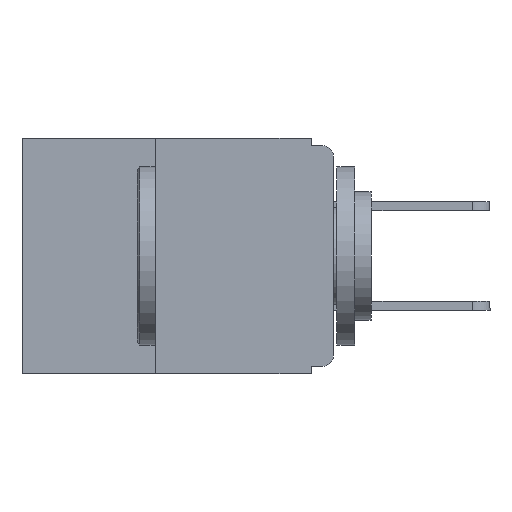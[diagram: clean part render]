
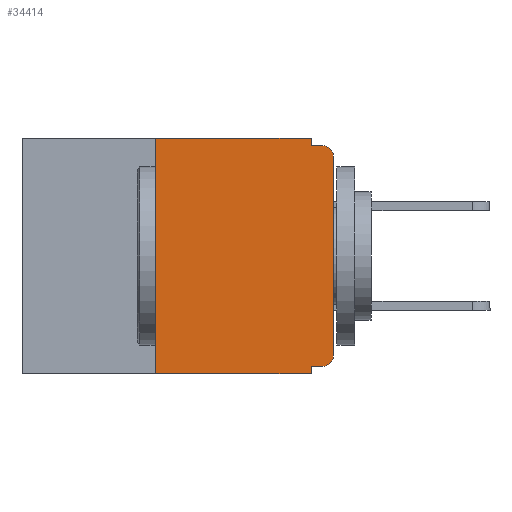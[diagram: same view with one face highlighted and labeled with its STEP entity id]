
A CAD part, left-side view. The second image highlights one B-rep face of the part: STEP entity #34414.
In plain terms, the highlighted planar face has unit normal (-1, 0, 0).
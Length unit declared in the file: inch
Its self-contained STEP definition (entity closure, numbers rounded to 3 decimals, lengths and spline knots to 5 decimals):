
#306 = EDGE_CURVE ( 'NONE', #34625, #32192, #23658, .T. ) ;
#329 = EDGE_CURVE ( 'NONE', #21040, #31015, #22812, .T. ) ;
#1522 = CARTESIAN_POINT ( 'NONE',  ( 0., 0.031, -0.33 ) ) ;
#1570 = LINE ( 'NONE', #31925, #3321 ) ;
#1593 = CARTESIAN_POINT ( 'NONE',  ( 0., 0.031, -0.32 ) ) ;
#1774 = VERTEX_POINT ( 'NONE', #35393 ) ;
#2307 = EDGE_CURVE ( 'NONE', #27736, #34625, #25643, .T. ) ;
#2591 = EDGE_CURVE ( 'NONE', #31015, #5357, #12139, .T. ) ;
#3321 = VECTOR ( 'NONE', #12739, 39.37008 ) ;
#3756 = EDGE_CURVE ( 'NONE', #27736, #18249, #9905, .T. ) ;
#4069 = DIRECTION ( 'NONE',  ( 0., 0., -1. ) ) ;
#4406 = CARTESIAN_POINT ( 'NONE',  ( 0., 0.031, 0. ) ) ;
#4643 = VECTOR ( 'NONE', #4069, 39.37008 ) ;
#4780 = CARTESIAN_POINT ( 'NONE',  ( 0., 0.015, -0.025 ) ) ;
#4988 = LINE ( 'NONE', #14108, #14281 ) ;
#5357 = VERTEX_POINT ( 'NONE', #24695 ) ;
#5406 = ORIENTED_EDGE ( 'NONE', *, *, #29477, .F. ) ;
#5520 = ORIENTED_EDGE ( 'NONE', *, *, #2591, .F. ) ;
#6437 = LINE ( 'NONE', #18262, #19609 ) ;
#6829 = EDGE_LOOP ( 'NONE', ( #11845, #20843, #5406, #5520, #16899, #6907, #9740, #11984, #7380, #9985 ) ) ;
#6907 = ORIENTED_EDGE ( 'NONE', *, *, #18470, .F. ) ;
#7191 = VERTEX_POINT ( 'NONE', #8021 ) ;
#7380 = ORIENTED_EDGE ( 'NONE', *, *, #2307, .F. ) ;
#7490 = CARTESIAN_POINT ( 'NONE',  ( 0., 0., -0.305 ) ) ;
#7656 = DIRECTION ( 'NONE',  ( 0., 0., -1. ) ) ;
#8021 = CARTESIAN_POINT ( 'NONE',  ( 0., 0.25, -0.33 ) ) ;
#8043 = VECTOR ( 'NONE', #30868, 39.37008 ) ;
#8484 = VECTOR ( 'NONE', #18605, 39.37008 ) ;
#8785 = CARTESIAN_POINT ( 'NONE',  ( 0., 0.015, -0.01 ) ) ;
#9183 = DIRECTION ( 'NONE',  ( 1., 0., 0. ) ) ;
#9740 = ORIENTED_EDGE ( 'NONE', *, *, #14223, .T. ) ;
#9905 = CIRCLE ( 'NONE', #34007, 0.015 ) ;
#9985 = ORIENTED_EDGE ( 'NONE', *, *, #3756, .T. ) ;
#10740 = CIRCLE ( 'NONE', #24290, 0.015 ) ;
#11845 = ORIENTED_EDGE ( 'NONE', *, *, #24388, .T. ) ;
#11984 = ORIENTED_EDGE ( 'NONE', *, *, #306, .F. ) ;
#12139 = LINE ( 'NONE', #4406, #4643 ) ;
#12739 = DIRECTION ( 'NONE',  ( 0., -1., 0. ) ) ;
#14108 = CARTESIAN_POINT ( 'NONE',  ( 0., 0.25, -0.33 ) ) ;
#14223 = EDGE_CURVE ( 'NONE', #7191, #32192, #1570, .T. ) ;
#14281 = VECTOR ( 'NONE', #27779, 39.37008 ) ;
#16899 = ORIENTED_EDGE ( 'NONE', *, *, #329, .F. ) ;
#18249 = VERTEX_POINT ( 'NONE', #7490 ) ;
#18262 = CARTESIAN_POINT ( 'NONE',  ( 0., 0., 0. ) ) ;
#18455 = VECTOR ( 'NONE', #34443, 39.37008 ) ;
#18470 = EDGE_CURVE ( 'NONE', #7191, #21040, #4988, .T. ) ;
#18497 = CARTESIAN_POINT ( 'NONE',  ( 0., 0., -0.01 ) ) ;
#18605 = DIRECTION ( 'NONE',  ( 0., -1., 0. ) ) ;
#19231 = VERTEX_POINT ( 'NONE', #8785 ) ;
#19609 = VECTOR ( 'NONE', #34440, 39.37008 ) ;
#20262 = CARTESIAN_POINT ( 'NONE',  ( 0., 0.437, 0. ) ) ;
#20365 = FACE_OUTER_BOUND ( 'NONE', #6829, .T. ) ;
#20843 = ORIENTED_EDGE ( 'NONE', *, *, #34682, .T. ) ;
#21040 = VERTEX_POINT ( 'NONE', #29490 ) ;
#22812 = LINE ( 'NONE', #31064, #8043 ) ;
#23658 = LINE ( 'NONE', #31224, #30909 ) ;
#24088 = CARTESIAN_POINT ( 'NONE',  ( 0., 0., -0.32 ) ) ;
#24248 = DIRECTION ( 'NONE',  ( -1., 0., 0. ) ) ;
#24290 = AXIS2_PLACEMENT_3D ( 'NONE', #4780, #24248, #7656 ) ;
#24388 = EDGE_CURVE ( 'NONE', #18249, #1774, #6437, .T. ) ;
#24695 = CARTESIAN_POINT ( 'NONE',  ( 0., 0.031, -0.01 ) ) ;
#25643 = LINE ( 'NONE', #24088, #18455 ) ;
#25710 = PLANE ( 'NONE',  #28653 ) ;
#25724 = CARTESIAN_POINT ( 'NONE',  ( 0., 0.031, 0. ) ) ;
#27736 = VERTEX_POINT ( 'NONE', #34772 ) ;
#27779 = DIRECTION ( 'NONE',  ( 0., 0., 1. ) ) ;
#28475 = DIRECTION ( 'NONE',  ( 0., 0., -1. ) ) ;
#28653 = AXIS2_PLACEMENT_3D ( 'NONE', #20262, #9183, #28475 ) ;
#29192 = DIRECTION ( 'NONE',  ( -1., 0., 0. ) ) ;
#29477 = EDGE_CURVE ( 'NONE', #5357, #19231, #30477, .T. ) ;
#29490 = CARTESIAN_POINT ( 'NONE',  ( 0., 0.25, 0. ) ) ;
#30477 = LINE ( 'NONE', #18497, #8484 ) ;
#30868 = DIRECTION ( 'NONE',  ( 0., -1., 0. ) ) ;
#30909 = VECTOR ( 'NONE', #31172, 39.37008 ) ;
#31015 = VERTEX_POINT ( 'NONE', #25724 ) ;
#31064 = CARTESIAN_POINT ( 'NONE',  ( 0., 0.437, 0. ) ) ;
#31172 = DIRECTION ( 'NONE',  ( 0., 0., -1. ) ) ;
#31224 = CARTESIAN_POINT ( 'NONE',  ( 0., 0.031, -0.33 ) ) ;
#31925 = CARTESIAN_POINT ( 'NONE',  ( 0., 0.437, -0.33 ) ) ;
#32192 = VERTEX_POINT ( 'NONE', #1522 ) ;
#33827 = CARTESIAN_POINT ( 'NONE',  ( 0., 0.015, -0.305 ) ) ;
#34007 = AXIS2_PLACEMENT_3D ( 'NONE', #33827, #29192, #34774 ) ;
#34414 = ADVANCED_FACE ( 'NONE', ( #20365 ), #25710, .F. ) ;
#34440 = DIRECTION ( 'NONE',  ( 0., 0., 1. ) ) ;
#34443 = DIRECTION ( 'NONE',  ( 0., 1., 0. ) ) ;
#34625 = VERTEX_POINT ( 'NONE', #1593 ) ;
#34682 = EDGE_CURVE ( 'NONE', #1774, #19231, #10740, .T. ) ;
#34772 = CARTESIAN_POINT ( 'NONE',  ( 0., 0.015, -0.32 ) ) ;
#34774 = DIRECTION ( 'NONE',  ( 0., 0., -1. ) ) ;
#35393 = CARTESIAN_POINT ( 'NONE',  ( 0., 0., -0.025 ) ) ;
